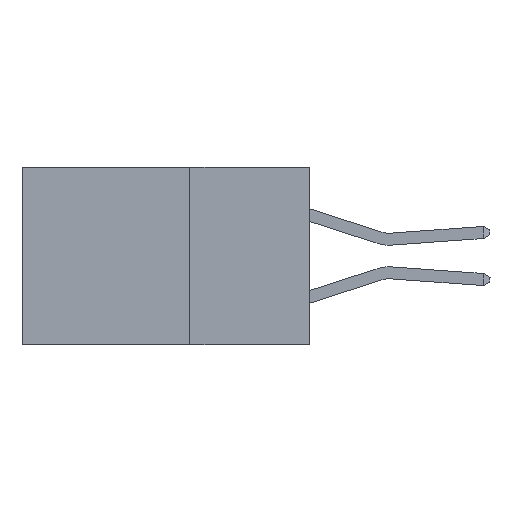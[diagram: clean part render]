
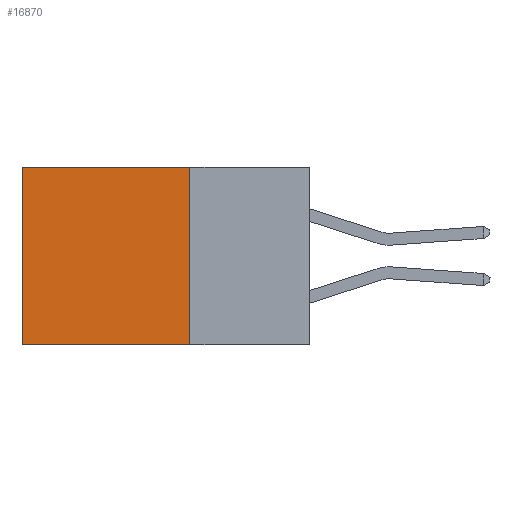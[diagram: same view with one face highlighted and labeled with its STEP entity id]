
A CAD part, left-side view. The second image highlights one B-rep face of the part: STEP entity #16870.
In plain terms, the highlighted planar face has unit normal (-1, 0, 0).
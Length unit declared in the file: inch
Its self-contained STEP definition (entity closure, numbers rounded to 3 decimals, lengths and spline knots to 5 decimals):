
#78 = DIRECTION ( 'NONE',  ( 0., 0., -1. ) ) ;
#115 = VERTEX_POINT ( 'NONE', #8641 ) ;
#938 = DIRECTION ( 'NONE',  ( 0., 0., -1. ) ) ;
#1033 = DIRECTION ( 'NONE',  ( 0., 0., -1. ) ) ;
#1313 = CARTESIAN_POINT ( 'NONE',  ( 0.2615, 0.25, 0. ) ) ;
#1385 = VERTEX_POINT ( 'NONE', #1313 ) ;
#2416 = CARTESIAN_POINT ( 'NONE',  ( 0.2615, 0.25, -0.37 ) ) ;
#2862 = LINE ( 'NONE', #4714, #14991 ) ;
#4405 = EDGE_LOOP ( 'NONE', ( #6094, #20229, #18256, #11695 ) ) ;
#4714 = CARTESIAN_POINT ( 'NONE',  ( 0.2615, 0.25, 0. ) ) ;
#4758 = CARTESIAN_POINT ( 'NONE',  ( 0.2615, 0.25, -0.37 ) ) ;
#5222 = CARTESIAN_POINT ( 'NONE',  ( 0.2615, 0.25, -0.37 ) ) ;
#6089 = EDGE_CURVE ( 'NONE', #1385, #20255, #12584, .T. ) ;
#6094 = ORIENTED_EDGE ( 'NONE', *, *, #11064, .T. ) ;
#6297 = DIRECTION ( 'NONE',  ( 0., 1., 0. ) ) ;
#7913 = PLANE ( 'NONE',  #8648 ) ;
#8297 = VECTOR ( 'NONE', #938, 39.37008 ) ;
#8641 = CARTESIAN_POINT ( 'NONE',  ( 0.2615, 0.6, -0.37 ) ) ;
#8648 = AXIS2_PLACEMENT_3D ( 'NONE', #4758, #9536, #78 ) ;
#9536 = DIRECTION ( 'NONE',  ( 1., 0., 0. ) ) ;
#10949 = CARTESIAN_POINT ( 'NONE',  ( 0.2615, 0.6, 0. ) ) ;
#11017 = LINE ( 'NONE', #2416, #14246 ) ;
#11064 = EDGE_CURVE ( 'NONE', #14640, #115, #15770, .T. ) ;
#11293 = EDGE_CURVE ( 'NONE', #1385, #14640, #2862, .T. ) ;
#11527 = VECTOR ( 'NONE', #1033, 39.37008 ) ;
#11695 = ORIENTED_EDGE ( 'NONE', *, *, #11293, .T. ) ;
#12123 = CARTESIAN_POINT ( 'NONE',  ( 0.2615, 0.6, -0.37 ) ) ;
#12584 = LINE ( 'NONE', #16749, #8297 ) ;
#14246 = VECTOR ( 'NONE', #19873, 39.37008 ) ;
#14640 = VERTEX_POINT ( 'NONE', #10949 ) ;
#14991 = VECTOR ( 'NONE', #6297, 39.37008 ) ;
#15770 = LINE ( 'NONE', #12123, #11527 ) ;
#16749 = CARTESIAN_POINT ( 'NONE',  ( 0.2615, 0.25, -0.37 ) ) ;
#16870 = ADVANCED_FACE ( 'NONE', ( #20246 ), #7913, .F. ) ;
#17211 = EDGE_CURVE ( 'NONE', #20255, #115, #11017, .T. ) ;
#18256 = ORIENTED_EDGE ( 'NONE', *, *, #6089, .F. ) ;
#19873 = DIRECTION ( 'NONE',  ( 0., 1., 0. ) ) ;
#20229 = ORIENTED_EDGE ( 'NONE', *, *, #17211, .F. ) ;
#20246 = FACE_OUTER_BOUND ( 'NONE', #4405, .T. ) ;
#20255 = VERTEX_POINT ( 'NONE', #5222 ) ;
